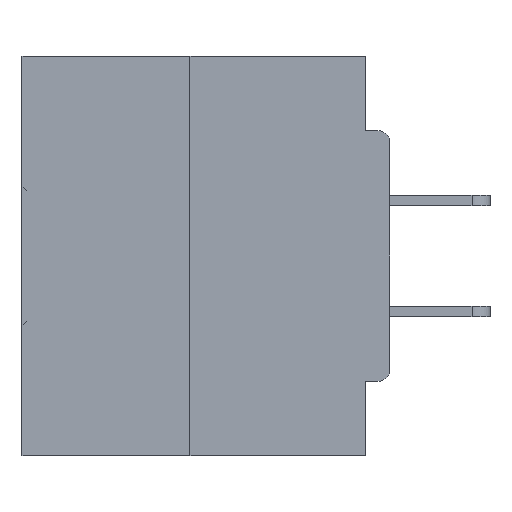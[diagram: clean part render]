
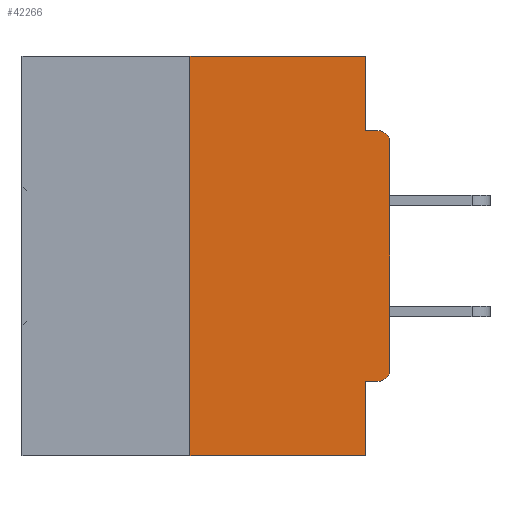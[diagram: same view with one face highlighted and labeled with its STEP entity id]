
A CAD part, left-side view. The second image highlights one B-rep face of the part: STEP entity #42266.
In plain terms, the highlighted planar face has unit normal (-1, 0, 0).
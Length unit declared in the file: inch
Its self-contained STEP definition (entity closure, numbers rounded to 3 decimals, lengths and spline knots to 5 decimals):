
#63 = ORIENTED_EDGE ( 'NONE', *, *, #292, .T. ) ;
#292 = EDGE_CURVE ( 'NONE', #12577, #27964, #6435, .T. ) ;
#597 = VERTEX_POINT ( 'NONE', #41164 ) ;
#1047 = CARTESIAN_POINT ( 'NONE',  ( 0., 0.015, -0.0935 ) ) ;
#1413 = LINE ( 'NONE', #8503, #23577 ) ;
#1694 = DIRECTION ( 'NONE',  ( -1., 0., 0. ) ) ;
#2332 = FACE_OUTER_BOUND ( 'NONE', #11658, .T. ) ;
#2639 = CARTESIAN_POINT ( 'NONE',  ( 0., 0.46, 0. ) ) ;
#2760 = CARTESIAN_POINT ( 'NONE',  ( 0., 0.015, -0.4065 ) ) ;
#2788 = PLANE ( 'NONE',  #15982 ) ;
#3920 = LINE ( 'NONE', #6948, #39691 ) ;
#4078 = CARTESIAN_POINT ( 'NONE',  ( 0., 0.031, 0. ) ) ;
#4510 = AXIS2_PLACEMENT_3D ( 'NONE', #15085, #4784, #18702 ) ;
#4784 = DIRECTION ( 'NONE',  ( -1., 0., 0. ) ) ;
#5146 = EDGE_CURVE ( 'NONE', #23796, #597, #6382, .T. ) ;
#5409 = CARTESIAN_POINT ( 'NONE',  ( 0., 0.46, 0. ) ) ;
#6382 = LINE ( 'NONE', #34859, #32951 ) ;
#6435 = CIRCLE ( 'NONE', #9314, 0.015 ) ;
#6901 = DIRECTION ( 'NONE',  ( 0., 0., 1. ) ) ;
#6948 = CARTESIAN_POINT ( 'NONE',  ( 0., 0., -0.0935 ) ) ;
#7100 = VERTEX_POINT ( 'NONE', #1047 ) ;
#7808 = DIRECTION ( 'NONE',  ( 0., -1., 0. ) ) ;
#8491 = DIRECTION ( 'NONE',  ( 0., 0., -1. ) ) ;
#8503 = CARTESIAN_POINT ( 'NONE',  ( 0., 0., 0. ) ) ;
#9314 = AXIS2_PLACEMENT_3D ( 'NONE', #29405, #1694, #8491 ) ;
#9744 = ORIENTED_EDGE ( 'NONE', *, *, #25423, .T. ) ;
#10184 = EDGE_CURVE ( 'NONE', #27716, #23434, #33833, .T. ) ;
#11658 = EDGE_LOOP ( 'NONE', ( #22074, #22611, #33086, #25133, #26328, #63, #9744, #42673, #28173, #39991 ) ) ;
#11837 = LINE ( 'NONE', #5409, #18854 ) ;
#12577 = VERTEX_POINT ( 'NONE', #2760 ) ;
#12769 = DIRECTION ( 'NONE',  ( 0., 0., -1. ) ) ;
#12849 = LINE ( 'NONE', #21411, #33481 ) ;
#15085 = CARTESIAN_POINT ( 'NONE',  ( 0., 0.015, -0.1085 ) ) ;
#15251 = VERTEX_POINT ( 'NONE', #35787 ) ;
#15982 = AXIS2_PLACEMENT_3D ( 'NONE', #2639, #26861, #12769 ) ;
#18654 = CIRCLE ( 'NONE', #4510, 0.015 ) ;
#18702 = DIRECTION ( 'NONE',  ( 0., 0., -1. ) ) ;
#18854 = VECTOR ( 'NONE', #22783, 39.37008 ) ;
#19495 = CARTESIAN_POINT ( 'NONE',  ( 0., 0.25, -0.5 ) ) ;
#19980 = CARTESIAN_POINT ( 'NONE',  ( 0., 0., -0.1085 ) ) ;
#20742 = VERTEX_POINT ( 'NONE', #21799 ) ;
#20859 = DIRECTION ( 'NONE',  ( 0., 0., -1. ) ) ;
#21253 = DIRECTION ( 'NONE',  ( 0., -1., 0. ) ) ;
#21411 = CARTESIAN_POINT ( 'NONE',  ( 0., 0., -0.4065 ) ) ;
#21799 = CARTESIAN_POINT ( 'NONE',  ( 0., 0.031, -0.4065 ) ) ;
#22074 = ORIENTED_EDGE ( 'NONE', *, *, #33714, .F. ) ;
#22611 = ORIENTED_EDGE ( 'NONE', *, *, #28393, .F. ) ;
#22783 = DIRECTION ( 'NONE',  ( 0., -1., 0. ) ) ;
#23434 = VERTEX_POINT ( 'NONE', #24119 ) ;
#23577 = VECTOR ( 'NONE', #36387, 39.37008 ) ;
#23796 = VERTEX_POINT ( 'NONE', #4078 ) ;
#24119 = CARTESIAN_POINT ( 'NONE',  ( 0., 0.031, -0.5 ) ) ;
#25133 = ORIENTED_EDGE ( 'NONE', *, *, #29577, .F. ) ;
#25296 = VECTOR ( 'NONE', #6901, 39.37008 ) ;
#25423 = EDGE_CURVE ( 'NONE', #27964, #44624, #1413, .T. ) ;
#25570 = EDGE_CURVE ( 'NONE', #44624, #7100, #18654, .T. ) ;
#26328 = ORIENTED_EDGE ( 'NONE', *, *, #28057, .F. ) ;
#26861 = DIRECTION ( 'NONE',  ( 1., 0., 0. ) ) ;
#27716 = VERTEX_POINT ( 'NONE', #19495 ) ;
#27964 = VERTEX_POINT ( 'NONE', #29521 ) ;
#28057 = EDGE_CURVE ( 'NONE', #12577, #20742, #12849, .T. ) ;
#28173 = ORIENTED_EDGE ( 'NONE', *, *, #31605, .F. ) ;
#28393 = EDGE_CURVE ( 'NONE', #27716, #15251, #31869, .T. ) ;
#29405 = CARTESIAN_POINT ( 'NONE',  ( 0., 0.015, -0.3915 ) ) ;
#29521 = CARTESIAN_POINT ( 'NONE',  ( 0., 0., -0.3915 ) ) ;
#29577 = EDGE_CURVE ( 'NONE', #20742, #23434, #30725, .T. ) ;
#30725 = LINE ( 'NONE', #38609, #44753 ) ;
#31605 = EDGE_CURVE ( 'NONE', #597, #7100, #3920, .T. ) ;
#31869 = LINE ( 'NONE', #44267, #25296 ) ;
#32951 = VECTOR ( 'NONE', #20859, 39.37008 ) ;
#33086 = ORIENTED_EDGE ( 'NONE', *, *, #10184, .T. ) ;
#33481 = VECTOR ( 'NONE', #42357, 39.37008 ) ;
#33714 = EDGE_CURVE ( 'NONE', #15251, #23796, #11837, .T. ) ;
#33833 = LINE ( 'NONE', #35829, #38688 ) ;
#34859 = CARTESIAN_POINT ( 'NONE',  ( 0., 0.031, 0. ) ) ;
#35787 = CARTESIAN_POINT ( 'NONE',  ( 0., 0.25, 0. ) ) ;
#35829 = CARTESIAN_POINT ( 'NONE',  ( 0., 0.46, -0.5 ) ) ;
#36387 = DIRECTION ( 'NONE',  ( 0., 0., 1. ) ) ;
#38609 = CARTESIAN_POINT ( 'NONE',  ( 0., 0.031, -0.5 ) ) ;
#38688 = VECTOR ( 'NONE', #7808, 39.37008 ) ;
#39691 = VECTOR ( 'NONE', #21253, 39.37008 ) ;
#39991 = ORIENTED_EDGE ( 'NONE', *, *, #5146, .F. ) ;
#41164 = CARTESIAN_POINT ( 'NONE',  ( 0., 0.031, -0.0935 ) ) ;
#42266 = ADVANCED_FACE ( 'NONE', ( #2332 ), #2788, .F. ) ;
#42357 = DIRECTION ( 'NONE',  ( 0., 1., 0. ) ) ;
#42544 = DIRECTION ( 'NONE',  ( 0., 0., -1. ) ) ;
#42673 = ORIENTED_EDGE ( 'NONE', *, *, #25570, .T. ) ;
#44267 = CARTESIAN_POINT ( 'NONE',  ( 0., 0.25, 0. ) ) ;
#44624 = VERTEX_POINT ( 'NONE', #19980 ) ;
#44753 = VECTOR ( 'NONE', #42544, 39.37008 ) ;
